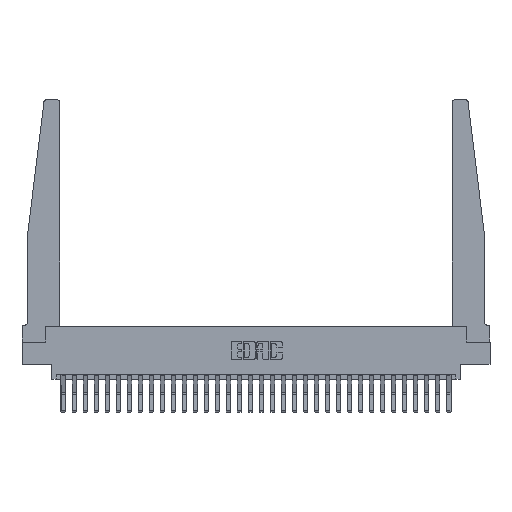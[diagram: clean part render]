
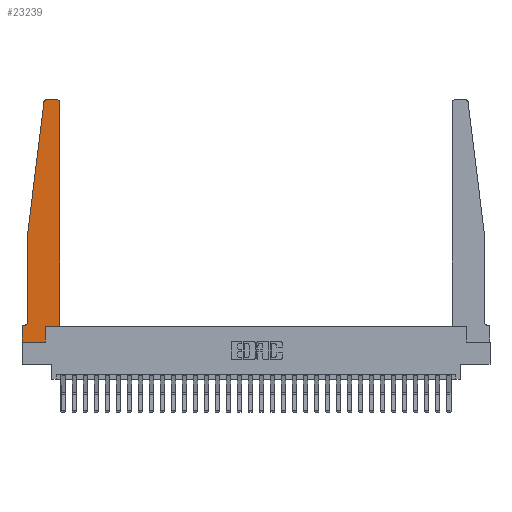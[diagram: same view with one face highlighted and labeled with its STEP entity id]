
A CAD part, top view. The second image highlights one B-rep face of the part: STEP entity #23239.
In plain terms, the highlighted planar face has unit normal (0, 0, 1).
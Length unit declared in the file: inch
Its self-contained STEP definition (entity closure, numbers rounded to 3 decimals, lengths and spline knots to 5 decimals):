
#262 = DIRECTION ( 'NONE',  ( 0., 0., 1. ) ) ;
#577 = EDGE_CURVE ( 'NONE', #28807, #13773, #12996, .T. ) ;
#869 = AXIS2_PLACEMENT_3D ( 'NONE', #6299, #22108, #8581 ) ;
#1572 = ORIENTED_EDGE ( 'NONE', *, *, #25040, .T. ) ;
#1708 = VECTOR ( 'NONE', #15322, 39.37008 ) ;
#1763 = AXIS2_PLACEMENT_3D ( 'NONE', #23304, #9784, #25577 ) ;
#1945 = CARTESIAN_POINT ( 'NONE',  ( 0., 0., 0.37 ) ) ;
#2229 = CARTESIAN_POINT ( 'NONE',  ( 0., 0.1875, 0.37 ) ) ;
#2866 = EDGE_LOOP ( 'NONE', ( #15840, #1572, #14454, #13948, #28770, #13622, #5598, #25051, #16274, #26946, #19890, #9977 ) ) ;
#2873 = VECTOR ( 'NONE', #12011, 39.37008 ) ;
#2923 = LINE ( 'NONE', #24593, #26265 ) ;
#2966 = CARTESIAN_POINT ( 'NONE',  ( 0.27653, 2.75, 0.37 ) ) ;
#3087 = VERTEX_POINT ( 'NONE', #27482 ) ;
#3133 = LINE ( 'NONE', #26560, #1708 ) ;
#3445 = VERTEX_POINT ( 'NONE', #24003 ) ;
#4055 = VERTEX_POINT ( 'NONE', #22524 ) ;
#4127 = CARTESIAN_POINT ( 'NONE',  ( 0.2605, 0.18, 0.37 ) ) ;
#4226 = DIRECTION ( 'NONE',  ( 0., -1., 0. ) ) ;
#4260 = FACE_OUTER_BOUND ( 'NONE', #2866, .T. ) ;
#4290 = LINE ( 'NONE', #5148, #2873 ) ;
#4366 = CIRCLE ( 'NONE', #10716, 0.03 ) ;
#4517 = DIRECTION ( 'NONE',  ( 1., 0., 0. ) ) ;
#4604 = VERTEX_POINT ( 'NONE', #26840 ) ;
#4808 = CARTESIAN_POINT ( 'NONE',  ( 0.065, 0.1875, 0.37 ) ) ;
#5148 = CARTESIAN_POINT ( 'NONE',  ( 0.425, 0.18, 0.37 ) ) ;
#5598 = ORIENTED_EDGE ( 'NONE', *, *, #21798, .T. ) ;
#5713 = CARTESIAN_POINT ( 'NONE',  ( 0.2605, 0., 0.37 ) ) ;
#5798 = AXIS2_PLACEMENT_3D ( 'NONE', #2229, #18078, #4517 ) ;
#5805 = VERTEX_POINT ( 'NONE', #19965 ) ;
#5941 = VERTEX_POINT ( 'NONE', #18089 ) ;
#6225 = VECTOR ( 'NONE', #9364, 39.37008 ) ;
#6299 = CARTESIAN_POINT ( 'NONE',  ( 0.27653, 2.72, 0.37 ) ) ;
#6329 = CARTESIAN_POINT ( 'NONE',  ( 0.425, 0.18, 0.37 ) ) ;
#6558 = VERTEX_POINT ( 'NONE', #13250 ) ;
#7093 = DIRECTION ( 'NONE',  ( -1., 0., 0. ) ) ;
#7553 = EDGE_CURVE ( 'NONE', #5805, #28807, #28283, .T. ) ;
#7798 = DIRECTION ( 'NONE',  ( 0., -1., 0. ) ) ;
#8581 = DIRECTION ( 'NONE',  ( 1., 0., 0. ) ) ;
#8756 = CARTESIAN_POINT ( 'NONE',  ( 0., 0., 0.37 ) ) ;
#9364 = DIRECTION ( 'NONE',  ( 0., 1., 0. ) ) ;
#9678 = LINE ( 'NONE', #1945, #26982 ) ;
#9757 = VERTEX_POINT ( 'NONE', #2966 ) ;
#9784 = DIRECTION ( 'NONE',  ( 0., 0., -1. ) ) ;
#9977 = ORIENTED_EDGE ( 'NONE', *, *, #21308, .T. ) ;
#10073 = LINE ( 'NONE', #27119, #25956 ) ;
#10276 = VECTOR ( 'NONE', #13336, 39.37008 ) ;
#10716 = AXIS2_PLACEMENT_3D ( 'NONE', #13888, #262, #16151 ) ;
#11424 = DIRECTION ( 'NONE',  ( 1., 0., 0. ) ) ;
#11577 = CIRCLE ( 'NONE', #1763, 0.05 ) ;
#12011 = DIRECTION ( 'NONE',  ( 0., 1., 0. ) ) ;
#12409 = EDGE_CURVE ( 'NONE', #5941, #28843, #23749, .T. ) ;
#12528 = CARTESIAN_POINT ( 'NONE',  ( 0.2605, 0.18, 0.37 ) ) ;
#12996 = LINE ( 'NONE', #12528, #6225 ) ;
#13250 = CARTESIAN_POINT ( 'NONE',  ( 0.015, 0.1875, 0.37 ) ) ;
#13336 = DIRECTION ( 'NONE',  ( 1., 0., 0. ) ) ;
#13622 = ORIENTED_EDGE ( 'NONE', *, *, #16625, .T. ) ;
#13773 = VERTEX_POINT ( 'NONE', #4127 ) ;
#13888 = CARTESIAN_POINT ( 'NONE',  ( 0.395, 2.72, 0.37 ) ) ;
#13948 = ORIENTED_EDGE ( 'NONE', *, *, #12409, .T. ) ;
#14454 = ORIENTED_EDGE ( 'NONE', *, *, #21819, .T. ) ;
#14537 = CARTESIAN_POINT ( 'NONE',  ( 0.065, 1.25, 0.37 ) ) ;
#15322 = DIRECTION ( 'NONE',  ( -1., 0., 0. ) ) ;
#15840 = ORIENTED_EDGE ( 'NONE', *, *, #18007, .T. ) ;
#16151 = DIRECTION ( 'NONE',  ( 1., 0., 0. ) ) ;
#16274 = ORIENTED_EDGE ( 'NONE', *, *, #577, .T. ) ;
#16625 = EDGE_CURVE ( 'NONE', #6558, #3087, #18441, .T. ) ;
#18007 = EDGE_CURVE ( 'NONE', #3445, #9757, #3133, .T. ) ;
#18078 = DIRECTION ( 'NONE',  ( 0., 0., 1. ) ) ;
#18089 = CARTESIAN_POINT ( 'NONE',  ( 0.065, 1.25, 0.37 ) ) ;
#18441 = LINE ( 'NONE', #4808, #24442 ) ;
#19890 = ORIENTED_EDGE ( 'NONE', *, *, #22798, .T. ) ;
#19965 = CARTESIAN_POINT ( 'NONE',  ( 0., 0., 0.37 ) ) ;
#20147 = EDGE_CURVE ( 'NONE', #28843, #6558, #11577, .T. ) ;
#21308 = EDGE_CURVE ( 'NONE', #4055, #3445, #4366, .T. ) ;
#21798 = EDGE_CURVE ( 'NONE', #3087, #5805, #9678, .T. ) ;
#21819 = EDGE_CURVE ( 'NONE', #4604, #5941, #2923, .T. ) ;
#21845 = CIRCLE ( 'NONE', #869, 0.03 ) ;
#22108 = DIRECTION ( 'NONE',  ( 0., 0., 1. ) ) ;
#22524 = CARTESIAN_POINT ( 'NONE',  ( 0.425, 2.72, 0.37 ) ) ;
#22798 = EDGE_CURVE ( 'NONE', #28345, #4055, #4290, .T. ) ;
#23239 = ADVANCED_FACE ( 'NONE', ( #4260 ), #27061, .T. ) ;
#23304 = CARTESIAN_POINT ( 'NONE',  ( 0.015, 0.2375, 0.37 ) ) ;
#23749 = LINE ( 'NONE', #14537, #29037 ) ;
#23901 = CARTESIAN_POINT ( 'NONE',  ( 0.065, 0.2375, 0.37 ) ) ;
#24003 = CARTESIAN_POINT ( 'NONE',  ( 0.395, 2.75, 0.37 ) ) ;
#24442 = VECTOR ( 'NONE', #7093, 39.37008 ) ;
#24593 = CARTESIAN_POINT ( 'NONE',  ( 0.065, 1.25, 0.37 ) ) ;
#25040 = EDGE_CURVE ( 'NONE', #9757, #4604, #21845, .T. ) ;
#25051 = ORIENTED_EDGE ( 'NONE', *, *, #7553, .T. ) ;
#25577 = DIRECTION ( 'NONE',  ( -1., 0., 0. ) ) ;
#25956 = VECTOR ( 'NONE', #11424, 39.37008 ) ;
#26265 = VECTOR ( 'NONE', #26870, 39.37008 ) ;
#26560 = CARTESIAN_POINT ( 'NONE',  ( 0.25, 2.75, 0.37 ) ) ;
#26840 = CARTESIAN_POINT ( 'NONE',  ( 0.24675, 2.72367, 0.37 ) ) ;
#26870 = DIRECTION ( 'NONE',  ( -0.122, -0.992, 0. ) ) ;
#26946 = ORIENTED_EDGE ( 'NONE', *, *, #27770, .T. ) ;
#26982 = VECTOR ( 'NONE', #4226, 39.37008 ) ;
#27061 = PLANE ( 'NONE',  #5798 ) ;
#27119 = CARTESIAN_POINT ( 'NONE',  ( 0.425, 0.18, 0.37 ) ) ;
#27482 = CARTESIAN_POINT ( 'NONE',  ( 0., 0.1875, 0.37 ) ) ;
#27770 = EDGE_CURVE ( 'NONE', #13773, #28345, #10073, .T. ) ;
#28283 = LINE ( 'NONE', #8756, #10276 ) ;
#28345 = VERTEX_POINT ( 'NONE', #6329 ) ;
#28770 = ORIENTED_EDGE ( 'NONE', *, *, #20147, .T. ) ;
#28807 = VERTEX_POINT ( 'NONE', #5713 ) ;
#28843 = VERTEX_POINT ( 'NONE', #23901 ) ;
#29037 = VECTOR ( 'NONE', #7798, 39.37008 ) ;
